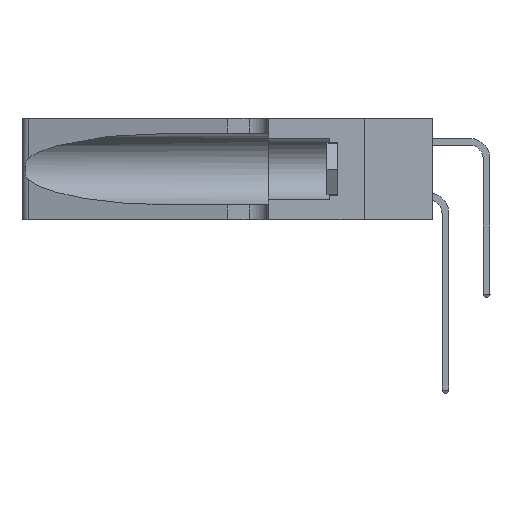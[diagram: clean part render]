
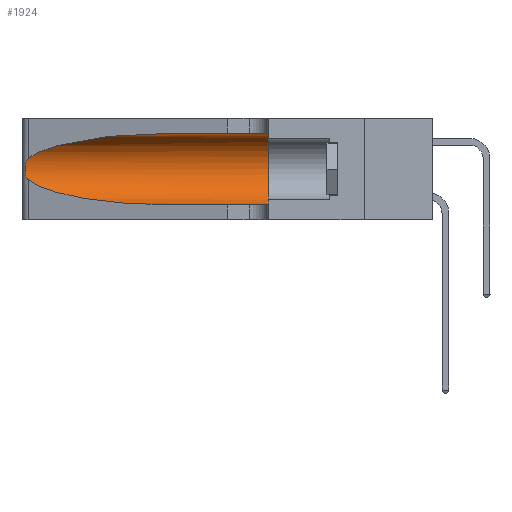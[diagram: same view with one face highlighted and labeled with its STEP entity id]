
A CAD part, left-side view. The second image highlights one B-rep face of the part: STEP entity #1924.
In plain terms, the highlighted cylindrical face has radius 3.308 mm (diameter 6.617 mm), a partial arc.
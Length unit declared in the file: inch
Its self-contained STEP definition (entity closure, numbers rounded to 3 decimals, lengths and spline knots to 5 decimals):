
#235 = EDGE_CURVE ( 'NONE', #29794, #18260, #29096, .T. ) ;
#1449 = CARTESIAN_POINT ( 'NONE',  ( 0.25854, 1.2359, 0.20912 ) ) ;
#1924 = ADVANCED_FACE ( 'NONE', ( #12560 ), #2401, .F. ) ;
#1992 = CARTESIAN_POINT ( 'NONE',  ( 0.26075, 1.23896, 0.19203 ) ) ;
#2400 = CARTESIAN_POINT ( 'NONE',  ( 0.2373, 1.15595, 0.28018 ) ) ;
#2401 = CYLINDRICAL_SURFACE ( 'NONE', #18429, 0.13025 ) ;
#3183 = EDGE_CURVE ( 'NONE', #32092, #34585, #8626, .T. ) ;
#3469 = CARTESIAN_POINT ( 'NONE',  ( 0.1305, 1.61858, 0.31525 ) ) ;
#3845 = CARTESIAN_POINT ( 'NONE',  ( 0.1305, 0.72297, 0.05475 ) ) ;
#4713 = CARTESIAN_POINT ( 'NONE',  ( 0.25789, 1.23486, 0.15765 ) ) ;
#4721 = ORIENTED_EDGE ( 'NONE', *, *, #3183, .T. ) ;
#4840 = CARTESIAN_POINT ( 'NONE',  ( 0.25487, 1.22718, 0.14631 ) ) ;
#5012 = ORIENTED_EDGE ( 'NONE', *, *, #34957, .T. ) ;
#5244 = VERTEX_POINT ( 'NONE', #24328 ) ;
#5974 = EDGE_LOOP ( 'NONE', ( #26974, #5012, #37248, #4721, #11042, #22199 ) ) ;
#7692 = CARTESIAN_POINT ( 'NONE',  ( 0.25856, 1.23593, 0.16098 ) ) ;
#8107 = CARTESIAN_POINT ( 'NONE',  ( 0.25639, 1.23184, 0.21858 ) ) ;
#8163 = CARTESIAN_POINT ( 'NONE',  ( 0.25487, 1.22718, 0.22369 ) ) ;
#8626 = LINE ( 'NONE', #19114, #22150 ) ;
#8896 = CARTESIAN_POINT ( 'NONE',  ( 0.1305, 0.72297, 0.31525 ) ) ;
#9490 = B_SPLINE_CURVE_WITH_KNOTS ( 'NONE', 3,
 ( #13779, #35415, #8107, #23378, #1449, #20500, #1992, #26610, #32689, #7692, #4713, #29713, #17114, #4840 ),
 .UNSPECIFIED., .F., .F.,
 ( 4, 2, 2, 2, 2, 2, 4 ),
 ( 0., 0.00027, 0.00053, 0.00107, 0.0016, 0.00187, 0.00214 ),
 .UNSPECIFIED. ) ;
#10142 = EDGE_CURVE ( 'NONE', #29794, #28577, #14674, .T. ) ;
#11042 = ORIENTED_EDGE ( 'NONE', *, *, #31047, .F. ) ;
#12560 = FACE_OUTER_BOUND ( 'NONE', #5974, .T. ) ;
#12572 = CARTESIAN_POINT ( 'NONE',  ( 0.1305, 0.35, 0.05475 ) ) ;
#13093 = AXIS2_PLACEMENT_3D ( 'NONE', #17624, #32929, #26857 ) ;
#13779 = CARTESIAN_POINT ( 'NONE',  ( 0.25487, 1.22718, 0.22369 ) ) ;
#14674 =( BOUNDED_CURVE ( )  B_SPLINE_CURVE ( 3, ( #8896, #30496, #2400, #30376 ),
 .UNSPECIFIED., .F., .T. ) 
 B_SPLINE_CURVE_WITH_KNOTS ( ( 4, 4 ),
 ( 1.5708, 2.84003 ),
 .UNSPECIFIED. ) 
 CURVE ( )  GEOMETRIC_REPRESENTATION_ITEM ( )  RATIONAL_B_SPLINE_CURVE ( ( 1., 0.87, 0.87, 1. ) ) 
 REPRESENTATION_ITEM ( '' )  );
#14812 = CARTESIAN_POINT ( 'NONE',  ( 0.1305, 1.61858, 0.185 ) ) ;
#16156 = DIRECTION ( 'NONE',  ( 0., -1., 0. ) ) ;
#16630 = CARTESIAN_POINT ( 'NONE',  ( 0.1305, 0.72297, 0.05475 ) ) ;
#17114 = CARTESIAN_POINT ( 'NONE',  ( 0.25555, 1.22993, 0.14849 ) ) ;
#17262 = CARTESIAN_POINT ( 'NONE',  ( 0.1305, 0.35, 0.31525 ) ) ;
#17624 = CARTESIAN_POINT ( 'NONE',  ( 0.1305, 0.35, 0.185 ) ) ;
#18260 = VERTEX_POINT ( 'NONE', #17262 ) ;
#18429 = AXIS2_PLACEMENT_3D ( 'NONE', #14812, #21917, #34644 ) ;
#19114 = CARTESIAN_POINT ( 'NONE',  ( 0.1305, 1.61858, 0.05475 ) ) ;
#20500 = CARTESIAN_POINT ( 'NONE',  ( 0.26018, 1.23835, 0.19895 ) ) ;
#21917 = DIRECTION ( 'NONE',  ( 0., -1., 0. ) ) ;
#22150 = VECTOR ( 'NONE', #16156, 39.37008 ) ;
#22199 = ORIENTED_EDGE ( 'NONE', *, *, #235, .F. ) ;
#22406 = DIRECTION ( 'NONE',  ( 0., -1., 0. ) ) ;
#22782 = CARTESIAN_POINT ( 'NONE',  ( 0.2373, 1.15595, 0.08982 ) ) ;
#23378 = CARTESIAN_POINT ( 'NONE',  ( 0.25787, 1.23484, 0.2124 ) ) ;
#24328 = CARTESIAN_POINT ( 'NONE',  ( 0.25487, 1.22718, 0.14631 ) ) ;
#25243 = VECTOR ( 'NONE', #22406, 39.37008 ) ;
#26610 = CARTESIAN_POINT ( 'NONE',  ( 0.26075, 1.23896, 0.178 ) ) ;
#26857 = DIRECTION ( 'NONE',  ( 0., 0., 1. ) ) ;
#26974 = ORIENTED_EDGE ( 'NONE', *, *, #10142, .T. ) ;
#28089 =( BOUNDED_CURVE ( )  B_SPLINE_CURVE ( 3, ( #38059, #22782, #34706, #3845 ),
 .UNSPECIFIED., .F., .T. ) 
 B_SPLINE_CURVE_WITH_KNOTS ( ( 4, 4 ),
 ( 3.44316, 4.71239 ),
 .UNSPECIFIED. ) 
 CURVE ( )  GEOMETRIC_REPRESENTATION_ITEM ( )  RATIONAL_B_SPLINE_CURVE ( ( 1., 0.87, 0.87, 1. ) ) 
 REPRESENTATION_ITEM ( '' )  );
#28577 = VERTEX_POINT ( 'NONE', #8163 ) ;
#29096 = LINE ( 'NONE', #3469, #25243 ) ;
#29694 = CARTESIAN_POINT ( 'NONE',  ( 0.1305, 0.72297, 0.31525 ) ) ;
#29713 = CARTESIAN_POINT ( 'NONE',  ( 0.25639, 1.23186, 0.15144 ) ) ;
#29794 = VERTEX_POINT ( 'NONE', #29694 ) ;
#30376 = CARTESIAN_POINT ( 'NONE',  ( 0.25487, 1.22718, 0.22369 ) ) ;
#30496 = CARTESIAN_POINT ( 'NONE',  ( 0.18966, 0.96281, 0.31525 ) ) ;
#31047 = EDGE_CURVE ( 'NONE', #18260, #34585, #31304, .T. ) ;
#31304 = CIRCLE ( 'NONE', #13093, 0.13025 ) ;
#32092 = VERTEX_POINT ( 'NONE', #16630 ) ;
#32689 = CARTESIAN_POINT ( 'NONE',  ( 0.26017, 1.23833, 0.17102 ) ) ;
#32929 = DIRECTION ( 'NONE',  ( 0., 1., 0. ) ) ;
#34585 = VERTEX_POINT ( 'NONE', #12572 ) ;
#34644 = DIRECTION ( 'NONE',  ( 0., 0., -1. ) ) ;
#34706 = CARTESIAN_POINT ( 'NONE',  ( 0.18966, 0.96281, 0.05475 ) ) ;
#34957 = EDGE_CURVE ( 'NONE', #28577, #5244, #9490, .T. ) ;
#35415 = CARTESIAN_POINT ( 'NONE',  ( 0.25555, 1.22994, 0.2215 ) ) ;
#37248 = ORIENTED_EDGE ( 'NONE', *, *, #39500, .T. ) ;
#38059 = CARTESIAN_POINT ( 'NONE',  ( 0.25487, 1.22718, 0.14631 ) ) ;
#39500 = EDGE_CURVE ( 'NONE', #5244, #32092, #28089, .T. ) ;
